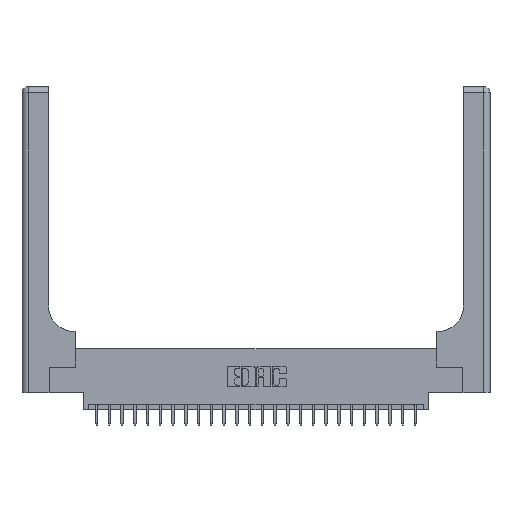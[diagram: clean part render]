
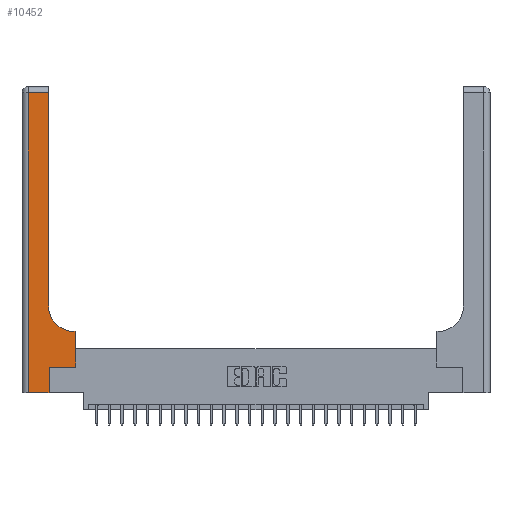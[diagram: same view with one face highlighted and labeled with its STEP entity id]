
A CAD part, top view. The second image highlights one B-rep face of the part: STEP entity #10452.
In plain terms, the highlighted planar face has unit normal (0, 0, 1).
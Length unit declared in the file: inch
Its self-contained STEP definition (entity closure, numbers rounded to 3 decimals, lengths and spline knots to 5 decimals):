
#416 = DIRECTION ( 'NONE',  ( -1., 0., 0. ) ) ;
#519 = VECTOR ( 'NONE', #16789, 39.37008 ) ;
#1300 = AXIS2_PLACEMENT_3D ( 'NONE', #24329, #5183, #12866 ) ;
#1557 = VERTEX_POINT ( 'NONE', #9672 ) ;
#1911 = ORIENTED_EDGE ( 'NONE', *, *, #5480, .T. ) ;
#2049 = VERTEX_POINT ( 'NONE', #2409 ) ;
#2120 = DIRECTION ( 'NONE',  ( -1., 0., 0. ) ) ;
#2311 = LINE ( 'NONE', #6230, #6164 ) ;
#2409 = CARTESIAN_POINT ( 'NONE',  ( 0.26, 2.94, 0.37 ) ) ;
#2560 = ORIENTED_EDGE ( 'NONE', *, *, #23540, .T. ) ;
#3903 = VERTEX_POINT ( 'NONE', #16509 ) ;
#4016 = DIRECTION ( 'NONE',  ( 1., 0., 0. ) ) ;
#4549 = ORIENTED_EDGE ( 'NONE', *, *, #15240, .T. ) ;
#5183 = DIRECTION ( 'NONE',  ( 0., 0., -1. ) ) ;
#5396 = VECTOR ( 'NONE', #4016, 39.37008 ) ;
#5480 = EDGE_CURVE ( 'NONE', #11280, #3903, #21519, .T. ) ;
#5569 = LINE ( 'NONE', #9619, #519 ) ;
#6164 = VECTOR ( 'NONE', #416, 39.37008 ) ;
#6200 = ORIENTED_EDGE ( 'NONE', *, *, #24007, .T. ) ;
#6230 = CARTESIAN_POINT ( 'NONE',  ( 0., 2.94, 0.37 ) ) ;
#7207 = CARTESIAN_POINT ( 'NONE',  ( 0.265, 0., 0.37 ) ) ;
#7530 = VECTOR ( 'NONE', #13905, 39.37008 ) ;
#9619 = CARTESIAN_POINT ( 'NONE',  ( 0.265, 0.25, 0.37 ) ) ;
#9672 = CARTESIAN_POINT ( 'NONE',  ( 0.528, 0.25, 0.37 ) ) ;
#9697 = VERTEX_POINT ( 'NONE', #17807 ) ;
#10452 = ADVANCED_FACE ( 'NONE', ( #22438 ), #24458, .F. ) ;
#11191 = DIRECTION ( 'NONE',  ( 0., 0., -1. ) ) ;
#11244 = DIRECTION ( 'NONE',  ( 0., 1., 0. ) ) ;
#11280 = VERTEX_POINT ( 'NONE', #22502 ) ;
#11365 = EDGE_CURVE ( 'NONE', #19712, #2049, #17910, .T. ) ;
#11714 = CARTESIAN_POINT ( 'NONE',  ( 0.265, 0.25, 0.37 ) ) ;
#11951 = CARTESIAN_POINT ( 'NONE',  ( 0., 0., 0.37 ) ) ;
#12047 = ORIENTED_EDGE ( 'NONE', *, *, #13195, .T. ) ;
#12128 = ORIENTED_EDGE ( 'NONE', *, *, #22152, .T. ) ;
#12608 = DIRECTION ( 'NONE',  ( 0., 1., 0. ) ) ;
#12864 = LINE ( 'NONE', #7207, #18891 ) ;
#12866 = DIRECTION ( 'NONE',  ( -1., 0., 0. ) ) ;
#13065 = VECTOR ( 'NONE', #13182, 39.37008 ) ;
#13123 = EDGE_LOOP ( 'NONE', ( #15285, #4549, #12047, #1911, #16622, #2560, #12128, #6200, #18482 ) ) ;
#13182 = DIRECTION ( 'NONE',  ( 0., 1., 0. ) ) ;
#13195 = EDGE_CURVE ( 'NONE', #19782, #11280, #17665, .T. ) ;
#13905 = DIRECTION ( 'NONE',  ( 0., -1., 0. ) ) ;
#14046 = CARTESIAN_POINT ( 'NONE',  ( 0.06, 2.94, 0.37 ) ) ;
#14319 = CIRCLE ( 'NONE', #15148, 0.25 ) ;
#14530 = EDGE_CURVE ( 'NONE', #9697, #19712, #14319, .T. ) ;
#15148 = AXIS2_PLACEMENT_3D ( 'NONE', #20750, #11191, #20616 ) ;
#15240 = EDGE_CURVE ( 'NONE', #2049, #19782, #2311, .T. ) ;
#15285 = ORIENTED_EDGE ( 'NONE', *, *, #11365, .T. ) ;
#16509 = CARTESIAN_POINT ( 'NONE',  ( 0.265, 0., 0.37 ) ) ;
#16622 = ORIENTED_EDGE ( 'NONE', *, *, #16970, .T. ) ;
#16673 = VERTEX_POINT ( 'NONE', #22217 ) ;
#16789 = DIRECTION ( 'NONE',  ( 1., 0., 0. ) ) ;
#16970 = EDGE_CURVE ( 'NONE', #3903, #18971, #12864, .T. ) ;
#17497 = CARTESIAN_POINT ( 'NONE',  ( 0.26, 0.6, 0.37 ) ) ;
#17665 = LINE ( 'NONE', #19561, #7530 ) ;
#17807 = CARTESIAN_POINT ( 'NONE',  ( 0.51, 0.6, 0.37 ) ) ;
#17910 = LINE ( 'NONE', #21234, #13065 ) ;
#18482 = ORIENTED_EDGE ( 'NONE', *, *, #14530, .T. ) ;
#18891 = VECTOR ( 'NONE', #12608, 39.37008 ) ;
#18971 = VERTEX_POINT ( 'NONE', #11714 ) ;
#19084 = CARTESIAN_POINT ( 'NONE',  ( 0.26, 0.85, 0.37 ) ) ;
#19561 = CARTESIAN_POINT ( 'NONE',  ( 0.06, 3., 0.37 ) ) ;
#19712 = VERTEX_POINT ( 'NONE', #19084 ) ;
#19782 = VERTEX_POINT ( 'NONE', #14046 ) ;
#19861 = VECTOR ( 'NONE', #11244, 39.37008 ) ;
#20616 = DIRECTION ( 'NONE',  ( 1., 0., 0. ) ) ;
#20750 = CARTESIAN_POINT ( 'NONE',  ( 0.51, 0.85, 0.37 ) ) ;
#21234 = CARTESIAN_POINT ( 'NONE',  ( 0.26, 3., 0.37 ) ) ;
#21519 = LINE ( 'NONE', #11951, #5396 ) ;
#21652 = LINE ( 'NONE', #17497, #24688 ) ;
#22152 = EDGE_CURVE ( 'NONE', #1557, #16673, #24345, .T. ) ;
#22217 = CARTESIAN_POINT ( 'NONE',  ( 0.528, 0.6, 0.37 ) ) ;
#22438 = FACE_OUTER_BOUND ( 'NONE', #13123, .T. ) ;
#22502 = CARTESIAN_POINT ( 'NONE',  ( 0.06, 0., 0.37 ) ) ;
#23540 = EDGE_CURVE ( 'NONE', #18971, #1557, #5569, .T. ) ;
#24007 = EDGE_CURVE ( 'NONE', #16673, #9697, #21652, .T. ) ;
#24329 = CARTESIAN_POINT ( 'NONE',  ( 0., 3., 0.37 ) ) ;
#24345 = LINE ( 'NONE', #24843, #19861 ) ;
#24458 = PLANE ( 'NONE',  #1300 ) ;
#24688 = VECTOR ( 'NONE', #2120, 39.37008 ) ;
#24843 = CARTESIAN_POINT ( 'NONE',  ( 0.528, 0.25, 0.37 ) ) ;
